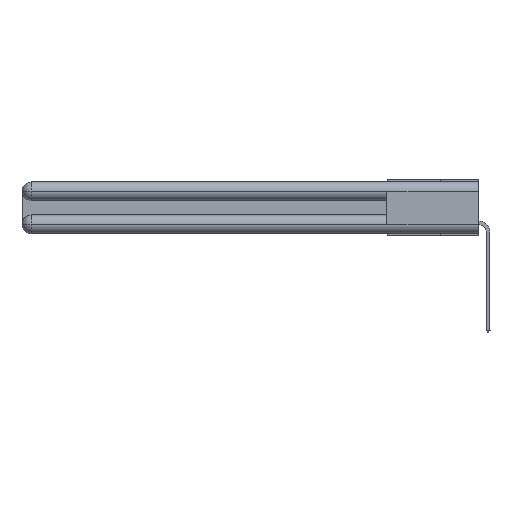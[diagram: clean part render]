
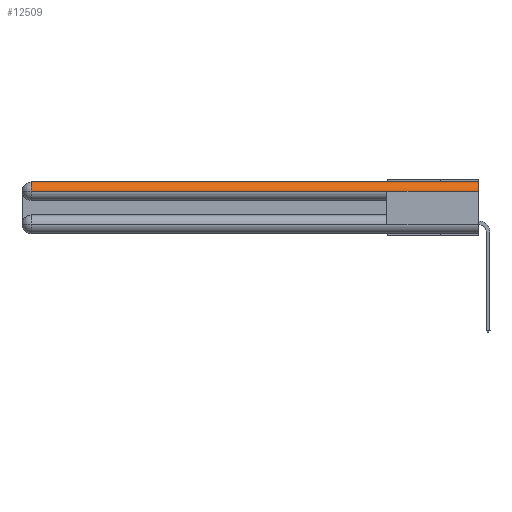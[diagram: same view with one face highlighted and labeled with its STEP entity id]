
A CAD part, left-side view. The second image highlights one B-rep face of the part: STEP entity #12509.
In plain terms, the highlighted cylindrical face has radius 1.562 mm (diameter 3.124 mm), a partial arc.
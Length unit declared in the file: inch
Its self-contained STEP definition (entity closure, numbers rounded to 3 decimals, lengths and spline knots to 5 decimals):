
#432 = ORIENTED_EDGE ( 'NONE', *, *, #25167, .F. ) ;
#838 = VERTEX_POINT ( 'NONE', #24859 ) ;
#2781 = DIRECTION ( 'NONE',  ( 0., 0., 1. ) ) ;
#4908 = EDGE_CURVE ( 'NONE', #18365, #8961, #25980, .T. ) ;
#5130 = VERTEX_POINT ( 'NONE', #12660 ) ;
#5140 = CARTESIAN_POINT ( 'NONE',  ( 0.0615, 2.94, -0.0615 ) ) ;
#5372 = FACE_OUTER_BOUND ( 'NONE', #22643, .T. ) ;
#5585 = DIRECTION ( 'NONE',  ( 0., 1., 0. ) ) ;
#7103 = DIRECTION ( 'NONE',  ( 0., 0., 1. ) ) ;
#7818 = CYLINDRICAL_SURFACE ( 'NONE', #15908, 0.0615 ) ;
#7961 = ORIENTED_EDGE ( 'NONE', *, *, #16559, .F. ) ;
#8860 = ORIENTED_EDGE ( 'NONE', *, *, #23674, .T. ) ;
#8961 = VERTEX_POINT ( 'NONE', #18103 ) ;
#9290 = AXIS2_PLACEMENT_3D ( 'NONE', #26561, #26456, #24202 ) ;
#11695 = CARTESIAN_POINT ( 'NONE',  ( 0., 0.6, -0.0615 ) ) ;
#12258 = AXIS2_PLACEMENT_3D ( 'NONE', #5140, #15988, #2781 ) ;
#12509 = ADVANCED_FACE ( 'NONE', ( #5372 ), #7818, .T. ) ;
#12660 = CARTESIAN_POINT ( 'NONE',  ( 0., 0., -0.0615 ) ) ;
#12751 = DIRECTION ( 'NONE',  ( 0., -1., 0. ) ) ;
#15037 = VERTEX_POINT ( 'NONE', #11695 ) ;
#15908 = AXIS2_PLACEMENT_3D ( 'NONE', #18278, #20534, #7103 ) ;
#15988 = DIRECTION ( 'NONE',  ( 0., -1., 0. ) ) ;
#16559 = EDGE_CURVE ( 'NONE', #5130, #15037, #24532, .T. ) ;
#18103 = CARTESIAN_POINT ( 'NONE',  ( 0.0615, 0., 0. ) ) ;
#18278 = CARTESIAN_POINT ( 'NONE',  ( 0.0615, 0., -0.0615 ) ) ;
#18365 = VERTEX_POINT ( 'NONE', #26027 ) ;
#20534 = DIRECTION ( 'NONE',  ( 0., 1., 0. ) ) ;
#21674 = VECTOR ( 'NONE', #12751, 39.37008 ) ;
#22643 = EDGE_LOOP ( 'NONE', ( #26485, #8860, #26551, #7961, #432 ) ) ;
#22836 = CARTESIAN_POINT ( 'NONE',  ( 0.0615, 0., 0. ) ) ;
#23379 = CARTESIAN_POINT ( 'NONE',  ( 0., 3., -0.0615 ) ) ;
#23674 = EDGE_CURVE ( 'NONE', #18365, #838, #27538, .T. ) ;
#23810 = CARTESIAN_POINT ( 'NONE',  ( 0., 3., -0.0615 ) ) ;
#24158 = VECTOR ( 'NONE', #5585, 39.37008 ) ;
#24202 = DIRECTION ( 'NONE',  ( 1., 0., 0. ) ) ;
#24532 = LINE ( 'NONE', #23379, #24158 ) ;
#24859 = CARTESIAN_POINT ( 'NONE',  ( 0., 2.94, -0.0615 ) ) ;
#25167 = EDGE_CURVE ( 'NONE', #8961, #5130, #28138, .T. ) ;
#25980 = LINE ( 'NONE', #22836, #27769 ) ;
#26027 = CARTESIAN_POINT ( 'NONE',  ( 0.0615, 2.94, 0. ) ) ;
#26456 = DIRECTION ( 'NONE',  ( 0., -1., 0. ) ) ;
#26485 = ORIENTED_EDGE ( 'NONE', *, *, #4908, .F. ) ;
#26551 = ORIENTED_EDGE ( 'NONE', *, *, #27014, .T. ) ;
#26561 = CARTESIAN_POINT ( 'NONE',  ( 0.0615, 0., -0.0615 ) ) ;
#27014 = EDGE_CURVE ( 'NONE', #838, #15037, #27663, .T. ) ;
#27405 = DIRECTION ( 'NONE',  ( 0., -1., 0. ) ) ;
#27538 = CIRCLE ( 'NONE', #12258, 0.0615 ) ;
#27663 = LINE ( 'NONE', #23810, #21674 ) ;
#27769 = VECTOR ( 'NONE', #27405, 39.37008 ) ;
#28138 = CIRCLE ( 'NONE', #9290, 0.0615 ) ;
